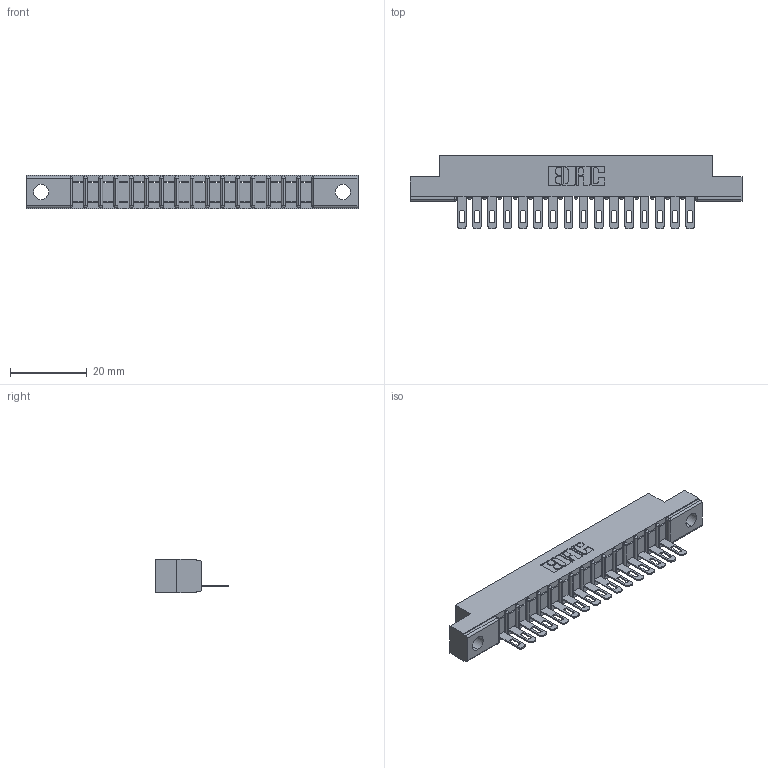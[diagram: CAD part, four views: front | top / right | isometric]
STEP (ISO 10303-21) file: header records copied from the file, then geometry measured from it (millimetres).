
FILE_DESCRIPTION (( 'STEP AP203' ), '1' );
FILE_NAME ('357-016-505-104.STEP', '2019-09-13T21:12:57', ( '' ), ( '' ), 'SwSTEP 2.0', 'SolidWorks 2016', '' );
FILE_SCHEMA (( 'CONFIG_CONTROL_DESIGN' ));
Length unit declared in the file: inch
Products named in the file (3): 307 Part_.156 Dia Mounting Holes; 307-290-001_505; 357-016-505-104
Assembly tree (17 placements, depth 2):
  357-016-505-104
    307 Part_.156 Dia Mounting Holes
    307-290-001_505  x16
Bounding box: 86.41 x 19.18 x 8.71 mm (x, y, z)
Volume: 5386.3 mm3; surface area: 8124.9 mm2
Topology: 17 solids, 17 shells, 1045 faces, 2951 edges, 1898 vertices
Faces by surface type: plane 660, cylinder 351, sphere 34
Entity records: 17314 total; most frequent: CARTESIAN_POINT 2910, ORIENTED_EDGE 2894, DIRECTION 2839, EDGE_CURVE 1447, VECTOR 1105, LINE 1105, VERTEX_POINT 938, AXIS2_PLACEMENT_3D 867
